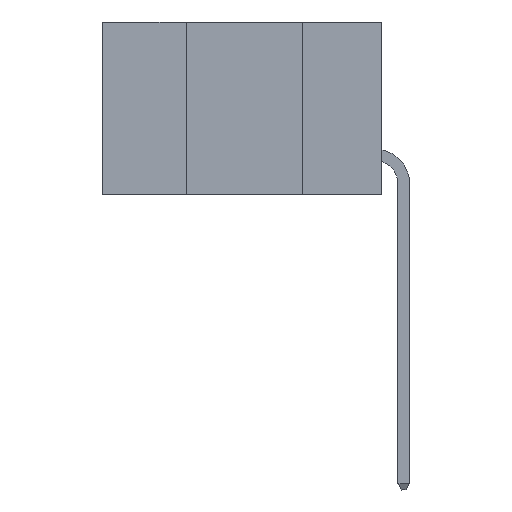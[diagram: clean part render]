
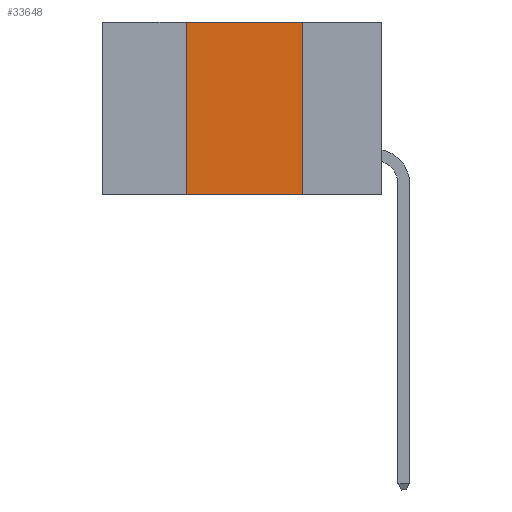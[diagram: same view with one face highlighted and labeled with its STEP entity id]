
A CAD part, left-side view. The second image highlights one B-rep face of the part: STEP entity #33648.
In plain terms, the highlighted planar face has unit normal (-1, 0, 0).
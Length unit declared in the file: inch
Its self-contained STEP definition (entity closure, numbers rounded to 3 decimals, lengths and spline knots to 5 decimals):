
#1680 = EDGE_LOOP ( 'NONE', ( #32930, #30941, #15278, #13549 ) ) ;
#3256 = CARTESIAN_POINT ( 'NONE',  ( 0., 0.42, 0. ) ) ;
#4711 = CARTESIAN_POINT ( 'NONE',  ( 0., 0.6, -0.37 ) ) ;
#4807 = LINE ( 'NONE', #30164, #19319 ) ;
#5424 = VECTOR ( 'NONE', #9521, 39.37008 ) ;
#6222 = CARTESIAN_POINT ( 'NONE',  ( 0., 0.6, 0. ) ) ;
#6481 = VERTEX_POINT ( 'NONE', #3256 ) ;
#9521 = DIRECTION ( 'NONE',  ( 0., -1., 0. ) ) ;
#10888 = VERTEX_POINT ( 'NONE', #41726 ) ;
#11197 = DIRECTION ( 'NONE',  ( 0., -1., 0. ) ) ;
#11364 = VECTOR ( 'NONE', #11197, 39.37008 ) ;
#13549 = ORIENTED_EDGE ( 'NONE', *, *, #37006, .T. ) ;
#14818 = CARTESIAN_POINT ( 'NONE',  ( 0., 0.6, 0. ) ) ;
#15278 = ORIENTED_EDGE ( 'NONE', *, *, #24968, .F. ) ;
#16084 = DIRECTION ( 'NONE',  ( 0., 0., -1. ) ) ;
#16214 = DIRECTION ( 'NONE',  ( 1., 0., 0. ) ) ;
#16403 = CARTESIAN_POINT ( 'NONE',  ( 0., 0.17, 0. ) ) ;
#16718 = DIRECTION ( 'NONE',  ( 0., 0., 1. ) ) ;
#18647 = CARTESIAN_POINT ( 'NONE',  ( 0., 0.42, -0.37 ) ) ;
#19319 = VECTOR ( 'NONE', #16718, 39.37008 ) ;
#20634 = VERTEX_POINT ( 'NONE', #18647 ) ;
#23652 = EDGE_CURVE ( 'NONE', #10888, #24165, #34945, .T. ) ;
#24165 = VERTEX_POINT ( 'NONE', #39539 ) ;
#24195 = EDGE_CURVE ( 'NONE', #6481, #10888, #40698, .T. ) ;
#24968 = EDGE_CURVE ( 'NONE', #20634, #6481, #4807, .T. ) ;
#30164 = CARTESIAN_POINT ( 'NONE',  ( 0., 0.42, 0. ) ) ;
#30449 = FACE_OUTER_BOUND ( 'NONE', #1680, .T. ) ;
#30941 = ORIENTED_EDGE ( 'NONE', *, *, #24195, .F. ) ;
#31948 = AXIS2_PLACEMENT_3D ( 'NONE', #14818, #16214, #16084 ) ;
#32930 = ORIENTED_EDGE ( 'NONE', *, *, #23652, .F. ) ;
#32988 = PLANE ( 'NONE',  #31948 ) ;
#33161 = LINE ( 'NONE', #4711, #11364 ) ;
#33419 = VECTOR ( 'NONE', #39592, 39.37008 ) ;
#33648 = ADVANCED_FACE ( 'NONE', ( #30449 ), #32988, .F. ) ;
#34945 = LINE ( 'NONE', #16403, #33419 ) ;
#37006 = EDGE_CURVE ( 'NONE', #20634, #24165, #33161, .T. ) ;
#39539 = CARTESIAN_POINT ( 'NONE',  ( 0., 0.17, -0.37 ) ) ;
#39592 = DIRECTION ( 'NONE',  ( 0., 0., -1. ) ) ;
#40698 = LINE ( 'NONE', #6222, #5424 ) ;
#41726 = CARTESIAN_POINT ( 'NONE',  ( 0., 0.17, 0. ) ) ;
